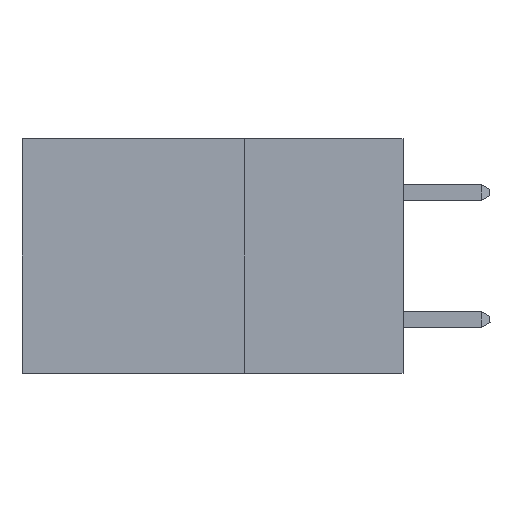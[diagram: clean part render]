
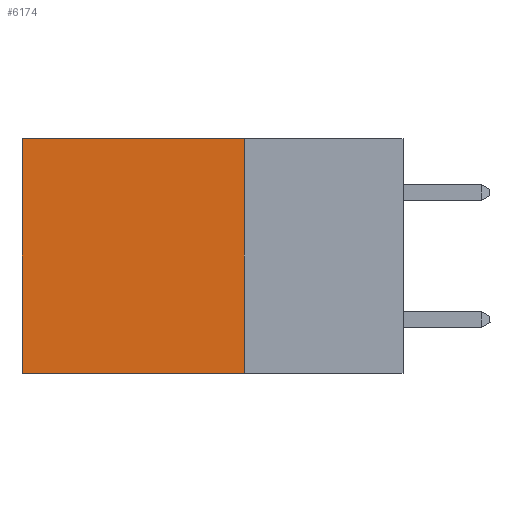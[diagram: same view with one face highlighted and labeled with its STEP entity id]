
A CAD part, left-side view. The second image highlights one B-rep face of the part: STEP entity #6174.
In plain terms, the highlighted planar face has unit normal (-1, 0, 0).
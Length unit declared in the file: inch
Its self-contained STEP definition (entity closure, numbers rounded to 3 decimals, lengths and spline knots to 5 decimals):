
#910 = CARTESIAN_POINT ( 'NONE',  ( 0.2875, 0.25, -0.37 ) ) ;
#1263 = DIRECTION ( 'NONE',  ( 0., 1., 0. ) ) ;
#1932 = LINE ( 'NONE', #8939, #15672 ) ;
#2972 = VERTEX_POINT ( 'NONE', #910 ) ;
#3186 = FACE_OUTER_BOUND ( 'NONE', #16281, .T. ) ;
#4442 = LINE ( 'NONE', #16742, #8552 ) ;
#6174 = ADVANCED_FACE ( 'NONE', ( #3186 ), #16300, .F. ) ;
#7376 = CARTESIAN_POINT ( 'NONE',  ( 0.2875, 0.25, 0. ) ) ;
#7718 = EDGE_CURVE ( 'NONE', #11837, #11703, #15966, .T. ) ;
#7727 = VERTEX_POINT ( 'NONE', #8452 ) ;
#7924 = EDGE_CURVE ( 'NONE', #2972, #7727, #1932, .T. ) ;
#8370 = CARTESIAN_POINT ( 'NONE',  ( 0.2875, 0.25, 0. ) ) ;
#8452 = CARTESIAN_POINT ( 'NONE',  ( 0.2875, 0.6, -0.37 ) ) ;
#8552 = VECTOR ( 'NONE', #18498, 39.37008 ) ;
#8939 = CARTESIAN_POINT ( 'NONE',  ( 0.2875, 0.25, -0.37 ) ) ;
#9181 = DIRECTION ( 'NONE',  ( 0., 0., -1. ) ) ;
#10548 = ORIENTED_EDGE ( 'NONE', *, *, #20220, .T. ) ;
#11262 = VECTOR ( 'NONE', #1263, 39.37008 ) ;
#11304 = LINE ( 'NONE', #20022, #20663 ) ;
#11703 = VERTEX_POINT ( 'NONE', #12644 ) ;
#11837 = VERTEX_POINT ( 'NONE', #16499 ) ;
#12407 = AXIS2_PLACEMENT_3D ( 'NONE', #7376, #19817, #9181 ) ;
#12644 = CARTESIAN_POINT ( 'NONE',  ( 0.2875, 0.6, 0. ) ) ;
#14892 = ORIENTED_EDGE ( 'NONE', *, *, #7924, .F. ) ;
#15016 = ORIENTED_EDGE ( 'NONE', *, *, #7718, .T. ) ;
#15672 = VECTOR ( 'NONE', #19685, 39.37008 ) ;
#15966 = LINE ( 'NONE', #8370, #11262 ) ;
#16281 = EDGE_LOOP ( 'NONE', ( #10548, #14892, #18348, #15016 ) ) ;
#16300 = PLANE ( 'NONE',  #12407 ) ;
#16499 = CARTESIAN_POINT ( 'NONE',  ( 0.2875, 0.25, 0. ) ) ;
#16674 = EDGE_CURVE ( 'NONE', #11837, #2972, #4442, .T. ) ;
#16742 = CARTESIAN_POINT ( 'NONE',  ( 0.2875, 0.25, 0. ) ) ;
#18348 = ORIENTED_EDGE ( 'NONE', *, *, #16674, .F. ) ;
#18498 = DIRECTION ( 'NONE',  ( 0., 0., -1. ) ) ;
#19685 = DIRECTION ( 'NONE',  ( 0., 1., 0. ) ) ;
#19817 = DIRECTION ( 'NONE',  ( 1., 0., 0. ) ) ;
#20022 = CARTESIAN_POINT ( 'NONE',  ( 0.2875, 0.6, 0. ) ) ;
#20220 = EDGE_CURVE ( 'NONE', #11703, #7727, #11304, .T. ) ;
#20663 = VECTOR ( 'NONE', #21748, 39.37008 ) ;
#21748 = DIRECTION ( 'NONE',  ( 0., 0., -1. ) ) ;
